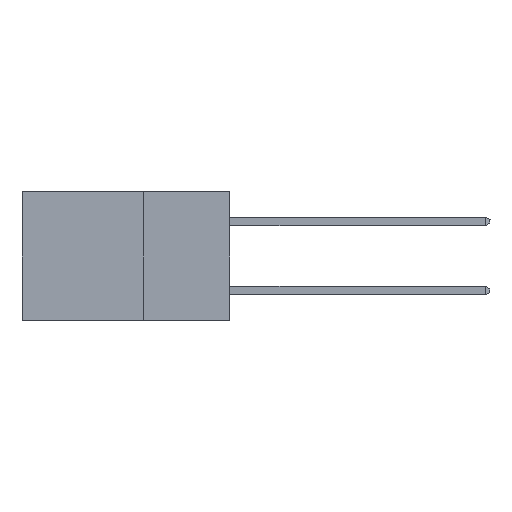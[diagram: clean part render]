
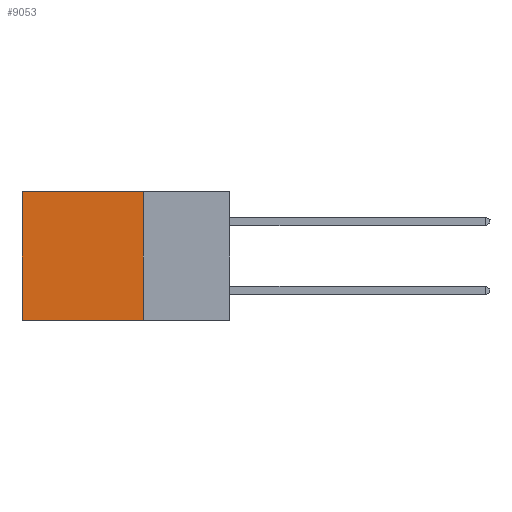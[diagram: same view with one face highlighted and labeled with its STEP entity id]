
A CAD part, left-side view. The second image highlights one B-rep face of the part: STEP entity #9053.
In plain terms, the highlighted planar face has unit normal (-1, 0, 0).
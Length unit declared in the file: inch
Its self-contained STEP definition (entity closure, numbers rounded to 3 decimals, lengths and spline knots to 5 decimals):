
#816 = VECTOR ( 'NONE', #1118, 39.37008 ) ;
#835 = DIRECTION ( 'NONE',  ( 1., 0., 0. ) ) ;
#1112 = DIRECTION ( 'NONE',  ( 0., 1., 0. ) ) ;
#1118 = DIRECTION ( 'NONE',  ( 0., 0., -1. ) ) ;
#1531 = EDGE_LOOP ( 'NONE', ( #1737, #13055, #2835, #13771 ) ) ;
#1589 = CARTESIAN_POINT ( 'NONE',  ( 0.2615, 0.6, 0. ) ) ;
#1737 = ORIENTED_EDGE ( 'NONE', *, *, #7920, .T. ) ;
#1832 = CARTESIAN_POINT ( 'NONE',  ( 0.2615, 0.25, -0.37 ) ) ;
#1980 = CARTESIAN_POINT ( 'NONE',  ( 0.2615, 0.25, 0. ) ) ;
#2835 = ORIENTED_EDGE ( 'NONE', *, *, #6757, .F. ) ;
#3970 = FACE_OUTER_BOUND ( 'NONE', #1531, .T. ) ;
#4106 = DIRECTION ( 'NONE',  ( 0., 0., -1. ) ) ;
#4120 = DIRECTION ( 'NONE',  ( 0., 1., 0. ) ) ;
#5131 = DIRECTION ( 'NONE',  ( 0., 0., -1. ) ) ;
#5591 = LINE ( 'NONE', #8576, #10005 ) ;
#5642 = AXIS2_PLACEMENT_3D ( 'NONE', #1832, #835, #4106 ) ;
#5815 = VECTOR ( 'NONE', #4120, 39.37008 ) ;
#5990 = CARTESIAN_POINT ( 'NONE',  ( 0.2615, 0.6, -0.37 ) ) ;
#6194 = LINE ( 'NONE', #12667, #10800 ) ;
#6757 = EDGE_CURVE ( 'NONE', #8906, #11575, #6194, .T. ) ;
#7196 = EDGE_CURVE ( 'NONE', #11575, #13404, #13840, .T. ) ;
#7920 = EDGE_CURVE ( 'NONE', #13174, #13404, #11989, .T. ) ;
#8576 = CARTESIAN_POINT ( 'NONE',  ( 0.2615, 0.25, 0. ) ) ;
#8906 = VERTEX_POINT ( 'NONE', #1980 ) ;
#9053 = ADVANCED_FACE ( 'NONE', ( #3970 ), #11564, .F. ) ;
#9262 = CARTESIAN_POINT ( 'NONE',  ( 0.2615, 0.25, -0.37 ) ) ;
#10005 = VECTOR ( 'NONE', #1112, 39.37008 ) ;
#10800 = VECTOR ( 'NONE', #5131, 39.37008 ) ;
#11318 = EDGE_CURVE ( 'NONE', #8906, #13174, #5591, .T. ) ;
#11564 = PLANE ( 'NONE',  #5642 ) ;
#11575 = VERTEX_POINT ( 'NONE', #12535 ) ;
#11989 = LINE ( 'NONE', #12910, #816 ) ;
#12535 = CARTESIAN_POINT ( 'NONE',  ( 0.2615, 0.25, -0.37 ) ) ;
#12667 = CARTESIAN_POINT ( 'NONE',  ( 0.2615, 0.25, -0.37 ) ) ;
#12910 = CARTESIAN_POINT ( 'NONE',  ( 0.2615, 0.6, -0.37 ) ) ;
#13055 = ORIENTED_EDGE ( 'NONE', *, *, #7196, .F. ) ;
#13174 = VERTEX_POINT ( 'NONE', #1589 ) ;
#13404 = VERTEX_POINT ( 'NONE', #5990 ) ;
#13771 = ORIENTED_EDGE ( 'NONE', *, *, #11318, .T. ) ;
#13840 = LINE ( 'NONE', #9262, #5815 ) ;
